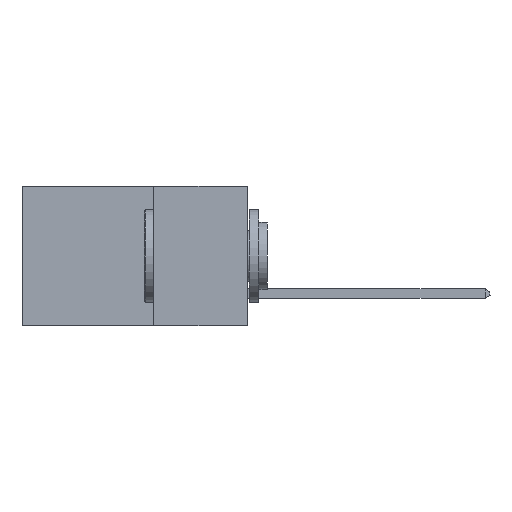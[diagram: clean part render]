
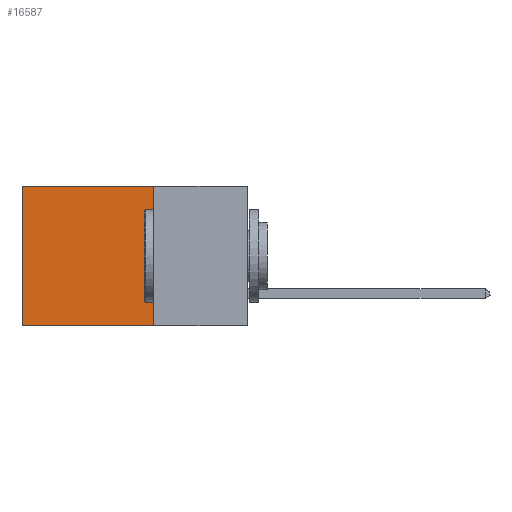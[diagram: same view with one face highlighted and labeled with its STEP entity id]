
A CAD part, left-side view. The second image highlights one B-rep face of the part: STEP entity #16587.
In plain terms, the highlighted planar face has unit normal (-1, 0, 0).
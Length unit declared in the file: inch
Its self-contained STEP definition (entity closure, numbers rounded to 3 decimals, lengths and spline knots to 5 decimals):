
#655 = VECTOR ( 'NONE', #9608, 39.37008 ) ;
#789 = CARTESIAN_POINT ( 'NONE',  ( 0.298, 0.25, 0. ) ) ;
#1227 = DIRECTION ( 'NONE',  ( 0., 0., -1. ) ) ;
#1762 = CARTESIAN_POINT ( 'NONE',  ( 0.298, 0.6, 0. ) ) ;
#1832 = VECTOR ( 'NONE', #1227, 39.37008 ) ;
#2535 = CARTESIAN_POINT ( 'NONE',  ( 0.298, 0.25, -0.37 ) ) ;
#3104 = ORIENTED_EDGE ( 'NONE', *, *, #11450, .F. ) ;
#4420 = LINE ( 'NONE', #2535, #655 ) ;
#4527 = ORIENTED_EDGE ( 'NONE', *, *, #6187, .F. ) ;
#5750 = DIRECTION ( 'NONE',  ( 0., 0., -1. ) ) ;
#6187 = EDGE_CURVE ( 'NONE', #9147, #15906, #11930, .T. ) ;
#6898 = CARTESIAN_POINT ( 'NONE',  ( 0.298, 0.6, -0.37 ) ) ;
#6935 = CARTESIAN_POINT ( 'NONE',  ( 0.298, 0.6, 0. ) ) ;
#7860 = CARTESIAN_POINT ( 'NONE',  ( 0.298, 0.25, -0.37 ) ) ;
#7919 = DIRECTION ( 'NONE',  ( 0., 1., 0. ) ) ;
#8494 = CARTESIAN_POINT ( 'NONE',  ( 0.298, 0.25, 0. ) ) ;
#8611 = PLANE ( 'NONE',  #13111 ) ;
#9042 = VECTOR ( 'NONE', #14712, 39.37008 ) ;
#9147 = VERTEX_POINT ( 'NONE', #17623 ) ;
#9381 = LINE ( 'NONE', #6935, #1832 ) ;
#9608 = DIRECTION ( 'NONE',  ( 0., 1., 0. ) ) ;
#9614 = FACE_OUTER_BOUND ( 'NONE', #12456, .T. ) ;
#10769 = VERTEX_POINT ( 'NONE', #1762 ) ;
#11105 = VERTEX_POINT ( 'NONE', #6898 ) ;
#11147 = VECTOR ( 'NONE', #7919, 39.37008 ) ;
#11208 = ORIENTED_EDGE ( 'NONE', *, *, #17743, .T. ) ;
#11374 = DIRECTION ( 'NONE',  ( 1., 0., 0. ) ) ;
#11450 = EDGE_CURVE ( 'NONE', #15906, #11105, #4420, .T. ) ;
#11930 = LINE ( 'NONE', #13279, #9042 ) ;
#12029 = LINE ( 'NONE', #789, #11147 ) ;
#12456 = EDGE_LOOP ( 'NONE', ( #13746, #3104, #4527, #11208 ) ) ;
#13111 = AXIS2_PLACEMENT_3D ( 'NONE', #8494, #11374, #5750 ) ;
#13279 = CARTESIAN_POINT ( 'NONE',  ( 0.298, 0.25, 0. ) ) ;
#13746 = ORIENTED_EDGE ( 'NONE', *, *, #14313, .T. ) ;
#14313 = EDGE_CURVE ( 'NONE', #10769, #11105, #9381, .T. ) ;
#14712 = DIRECTION ( 'NONE',  ( 0., 0., -1. ) ) ;
#15906 = VERTEX_POINT ( 'NONE', #7860 ) ;
#16587 = ADVANCED_FACE ( 'NONE', ( #9614 ), #8611, .F. ) ;
#17623 = CARTESIAN_POINT ( 'NONE',  ( 0.298, 0.25, 0. ) ) ;
#17743 = EDGE_CURVE ( 'NONE', #9147, #10769, #12029, .T. ) ;
